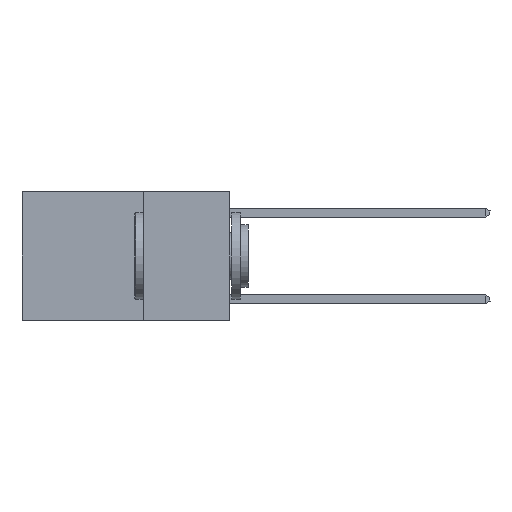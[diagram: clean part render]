
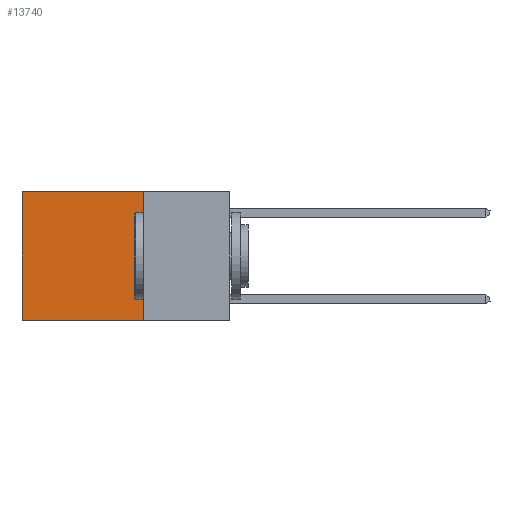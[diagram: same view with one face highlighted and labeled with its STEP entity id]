
A CAD part, left-side view. The second image highlights one B-rep face of the part: STEP entity #13740.
In plain terms, the highlighted planar face has unit normal (-1, 0, 0).
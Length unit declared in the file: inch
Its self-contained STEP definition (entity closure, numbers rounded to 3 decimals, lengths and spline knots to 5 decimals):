
#459 = ORIENTED_EDGE ( 'NONE', *, *, #6102, .F. ) ;
#990 = DIRECTION ( 'NONE',  ( 0., 1., 0. ) ) ;
#1253 = LINE ( 'NONE', #2461, #7228 ) ;
#1939 = CARTESIAN_POINT ( 'NONE',  ( 0.2625, 0.6, 0. ) ) ;
#2105 = DIRECTION ( 'NONE',  ( 0., 0., -1. ) ) ;
#2114 = CARTESIAN_POINT ( 'NONE',  ( 0.2625, 0.25, -0.37 ) ) ;
#2193 = DIRECTION ( 'NONE',  ( 0., 0., -1. ) ) ;
#2283 = VERTEX_POINT ( 'NONE', #9378 ) ;
#2461 = CARTESIAN_POINT ( 'NONE',  ( 0.2625, 0.25, 0. ) ) ;
#2705 = VERTEX_POINT ( 'NONE', #11484 ) ;
#3005 = EDGE_CURVE ( 'NONE', #14154, #2705, #7752, .T. ) ;
#3132 = VECTOR ( 'NONE', #990, 39.37008 ) ;
#3406 = LINE ( 'NONE', #4467, #11144 ) ;
#4461 = CARTESIAN_POINT ( 'NONE',  ( 0.2625, 0.25, 0. ) ) ;
#4467 = CARTESIAN_POINT ( 'NONE',  ( 0.2625, 0.25, 0. ) ) ;
#5081 = EDGE_LOOP ( 'NONE', ( #11751, #459, #6387, #14522 ) ) ;
#6102 = EDGE_CURVE ( 'NONE', #2283, #2705, #7791, .T. ) ;
#6387 = ORIENTED_EDGE ( 'NONE', *, *, #11838, .F. ) ;
#6783 = FACE_OUTER_BOUND ( 'NONE', #5081, .T. ) ;
#7228 = VECTOR ( 'NONE', #13121, 39.37008 ) ;
#7752 = LINE ( 'NONE', #1939, #9937 ) ;
#7791 = LINE ( 'NONE', #2114, #3132 ) ;
#9174 = VERTEX_POINT ( 'NONE', #4461 ) ;
#9378 = CARTESIAN_POINT ( 'NONE',  ( 0.2625, 0.25, -0.37 ) ) ;
#9803 = DIRECTION ( 'NONE',  ( 0., 0., -1. ) ) ;
#9937 = VECTOR ( 'NONE', #9803, 39.37008 ) ;
#10267 = PLANE ( 'NONE',  #13280 ) ;
#10999 = CARTESIAN_POINT ( 'NONE',  ( 0.2625, 0.6, 0. ) ) ;
#11010 = EDGE_CURVE ( 'NONE', #9174, #14154, #1253, .T. ) ;
#11144 = VECTOR ( 'NONE', #2193, 39.37008 ) ;
#11192 = DIRECTION ( 'NONE',  ( 1., 0., 0. ) ) ;
#11484 = CARTESIAN_POINT ( 'NONE',  ( 0.2625, 0.6, -0.37 ) ) ;
#11751 = ORIENTED_EDGE ( 'NONE', *, *, #3005, .T. ) ;
#11838 = EDGE_CURVE ( 'NONE', #9174, #2283, #3406, .T. ) ;
#12527 = CARTESIAN_POINT ( 'NONE',  ( 0.2625, 0.25, 0. ) ) ;
#13121 = DIRECTION ( 'NONE',  ( 0., 1., 0. ) ) ;
#13280 = AXIS2_PLACEMENT_3D ( 'NONE', #12527, #11192, #2105 ) ;
#13740 = ADVANCED_FACE ( 'NONE', ( #6783 ), #10267, .F. ) ;
#14154 = VERTEX_POINT ( 'NONE', #10999 ) ;
#14522 = ORIENTED_EDGE ( 'NONE', *, *, #11010, .T. ) ;
